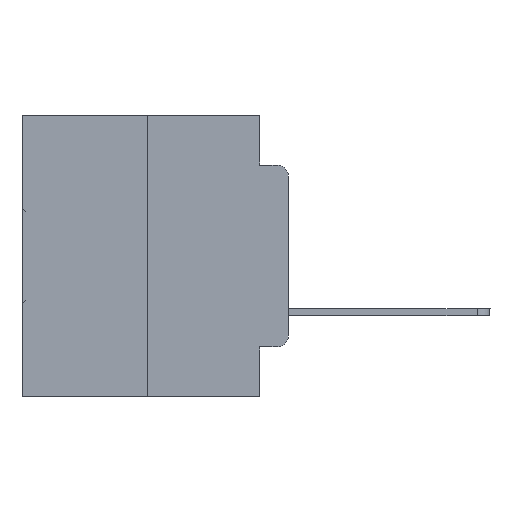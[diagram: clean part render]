
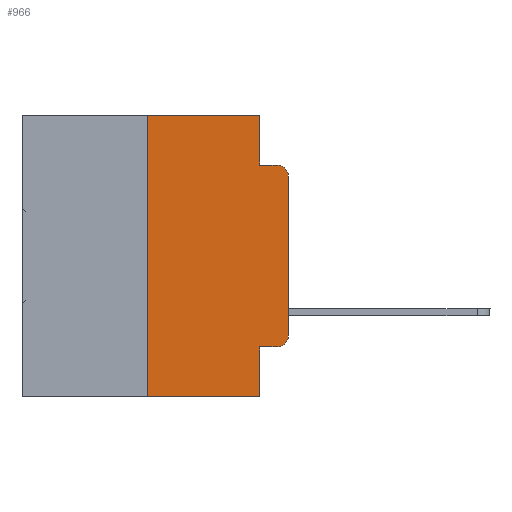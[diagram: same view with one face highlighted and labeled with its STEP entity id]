
A CAD part, left-side view. The second image highlights one B-rep face of the part: STEP entity #966.
In plain terms, the highlighted planar face has unit normal (-1, 0, 0).
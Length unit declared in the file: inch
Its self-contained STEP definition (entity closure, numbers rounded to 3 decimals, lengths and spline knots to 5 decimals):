
#112 = ORIENTED_EDGE ( 'NONE', *, *, #23995, .T. ) ;
#920 = VECTOR ( 'NONE', #23624, 39.37008 ) ;
#966 = ADVANCED_FACE ( 'NONE', ( #29396 ), #2952, .F. ) ;
#1161 = VECTOR ( 'NONE', #7430, 39.37008 ) ;
#1223 = VERTEX_POINT ( 'NONE', #29912 ) ;
#1409 = AXIS2_PLACEMENT_3D ( 'NONE', #13120, #25485, #3634 ) ;
#2000 = LINE ( 'NONE', #29377, #27557 ) ;
#2409 = CARTESIAN_POINT ( 'NONE',  ( 0., 0.25, 0. ) ) ;
#2458 = DIRECTION ( 'NONE',  ( -1., 0., 0. ) ) ;
#2721 = ORIENTED_EDGE ( 'NONE', *, *, #17437, .T. ) ;
#2754 = CARTESIAN_POINT ( 'NONE',  ( 0., 0.25, 0. ) ) ;
#2849 = CARTESIAN_POINT ( 'NONE',  ( 0., 0.473, 0. ) ) ;
#2899 = EDGE_CURVE ( 'NONE', #1223, #3802, #29334, .T. ) ;
#2952 = PLANE ( 'NONE',  #11335 ) ;
#3063 = DIRECTION ( 'NONE',  ( 0., 0., 1. ) ) ;
#3634 = DIRECTION ( 'NONE',  ( 0., 0., -1. ) ) ;
#3802 = VERTEX_POINT ( 'NONE', #2754 ) ;
#5614 = VERTEX_POINT ( 'NONE', #30076 ) ;
#6177 = EDGE_CURVE ( 'NONE', #16254, #25767, #12378, .T. ) ;
#6538 = CARTESIAN_POINT ( 'NONE',  ( 0., 0.051, -0.0885 ) ) ;
#7061 = LINE ( 'NONE', #28734, #12035 ) ;
#7262 = CARTESIAN_POINT ( 'NONE',  ( 0., 0.02, -0.3915 ) ) ;
#7430 = DIRECTION ( 'NONE',  ( 0., -1., 0. ) ) ;
#8000 = CARTESIAN_POINT ( 'NONE',  ( 0., 0., 0. ) ) ;
#9106 = EDGE_CURVE ( 'NONE', #31062, #9391, #9989, .T. ) ;
#9331 = ORIENTED_EDGE ( 'NONE', *, *, #30141, .F. ) ;
#9391 = VERTEX_POINT ( 'NONE', #18485 ) ;
#9632 = CARTESIAN_POINT ( 'NONE',  ( 0., 0., -0.3915 ) ) ;
#9983 = ORIENTED_EDGE ( 'NONE', *, *, #9106, .T. ) ;
#9989 = LINE ( 'NONE', #24395, #1161 ) ;
#10152 = DIRECTION ( 'NONE',  ( 0., 0., -1. ) ) ;
#11181 = CARTESIAN_POINT ( 'NONE',  ( 0., 0., -0.1085 ) ) ;
#11335 = AXIS2_PLACEMENT_3D ( 'NONE', #2849, #27047, #17357 ) ;
#11986 = VECTOR ( 'NONE', #27375, 39.37008 ) ;
#12035 = VECTOR ( 'NONE', #16607, 39.37008 ) ;
#12378 = CIRCLE ( 'NONE', #1409, 0.02 ) ;
#12832 = CARTESIAN_POINT ( 'NONE',  ( 0., 0.051, 0. ) ) ;
#12867 = ORIENTED_EDGE ( 'NONE', *, *, #2899, .F. ) ;
#12878 = CARTESIAN_POINT ( 'NONE',  ( 0., 0.051, 0. ) ) ;
#12962 = LINE ( 'NONE', #8000, #16401 ) ;
#13006 = CARTESIAN_POINT ( 'NONE',  ( 0., 0.473, 0. ) ) ;
#13120 = CARTESIAN_POINT ( 'NONE',  ( 0., 0.02, -0.1085 ) ) ;
#13848 = ORIENTED_EDGE ( 'NONE', *, *, #25305, .T. ) ;
#14674 = DIRECTION ( 'NONE',  ( 0., 0., 1. ) ) ;
#15008 = AXIS2_PLACEMENT_3D ( 'NONE', #7262, #2458, #24337 ) ;
#15818 = VERTEX_POINT ( 'NONE', #26516 ) ;
#16254 = VERTEX_POINT ( 'NONE', #11181 ) ;
#16401 = VECTOR ( 'NONE', #3063, 39.37008 ) ;
#16607 = DIRECTION ( 'NONE',  ( 0., 0., -1. ) ) ;
#16817 = CARTESIAN_POINT ( 'NONE',  ( 0., 0.02, -0.0885 ) ) ;
#17236 = DIRECTION ( 'NONE',  ( 0., -1., 0. ) ) ;
#17357 = DIRECTION ( 'NONE',  ( 0., 0., -1. ) ) ;
#17437 = EDGE_CURVE ( 'NONE', #9391, #30083, #25323, .T. ) ;
#18124 = VERTEX_POINT ( 'NONE', #12878 ) ;
#18485 = CARTESIAN_POINT ( 'NONE',  ( 0., 0.02, -0.4115 ) ) ;
#19222 = ORIENTED_EDGE ( 'NONE', *, *, #6177, .T. ) ;
#20436 = LINE ( 'NONE', #12832, #27624 ) ;
#20787 = LINE ( 'NONE', #13006, #11986 ) ;
#21011 = CARTESIAN_POINT ( 'NONE',  ( 0., 0.051, -0.4115 ) ) ;
#23624 = DIRECTION ( 'NONE',  ( 0., -1., 0. ) ) ;
#23995 = EDGE_CURVE ( 'NONE', #1223, #5614, #2000, .T. ) ;
#24337 = DIRECTION ( 'NONE',  ( 0., 0., -1. ) ) ;
#24392 = VECTOR ( 'NONE', #14674, 39.37008 ) ;
#24395 = CARTESIAN_POINT ( 'NONE',  ( 0., 0.051, -0.4115 ) ) ;
#24545 = ORIENTED_EDGE ( 'NONE', *, *, #29333, .F. ) ;
#25305 = EDGE_CURVE ( 'NONE', #30083, #16254, #12962, .T. ) ;
#25323 = CIRCLE ( 'NONE', #15008, 0.02 ) ;
#25485 = DIRECTION ( 'NONE',  ( -1., 0., 0. ) ) ;
#25767 = VERTEX_POINT ( 'NONE', #16817 ) ;
#26516 = CARTESIAN_POINT ( 'NONE',  ( 0., 0.051, -0.0885 ) ) ;
#27047 = DIRECTION ( 'NONE',  ( 1., 0., 0. ) ) ;
#27256 = LINE ( 'NONE', #6538, #920 ) ;
#27375 = DIRECTION ( 'NONE',  ( 0., -1., 0. ) ) ;
#27557 = VECTOR ( 'NONE', #17236, 39.37008 ) ;
#27624 = VECTOR ( 'NONE', #10152, 39.37008 ) ;
#28681 = EDGE_CURVE ( 'NONE', #18124, #15818, #7061, .T. ) ;
#28734 = CARTESIAN_POINT ( 'NONE',  ( 0., 0.051, 0. ) ) ;
#29333 = EDGE_CURVE ( 'NONE', #15818, #25767, #27256, .T. ) ;
#29334 = LINE ( 'NONE', #2409, #24392 ) ;
#29377 = CARTESIAN_POINT ( 'NONE',  ( 0., 0.473, -0.5 ) ) ;
#29396 = FACE_OUTER_BOUND ( 'NONE', #31573, .T. ) ;
#29471 = EDGE_CURVE ( 'NONE', #31062, #5614, #20436, .T. ) ;
#29912 = CARTESIAN_POINT ( 'NONE',  ( 0., 0.25, -0.5 ) ) ;
#30076 = CARTESIAN_POINT ( 'NONE',  ( 0., 0.051, -0.5 ) ) ;
#30083 = VERTEX_POINT ( 'NONE', #9632 ) ;
#30141 = EDGE_CURVE ( 'NONE', #3802, #18124, #20787, .T. ) ;
#30430 = ORIENTED_EDGE ( 'NONE', *, *, #28681, .F. ) ;
#30435 = ORIENTED_EDGE ( 'NONE', *, *, #29471, .F. ) ;
#31062 = VERTEX_POINT ( 'NONE', #21011 ) ;
#31573 = EDGE_LOOP ( 'NONE', ( #13848, #19222, #24545, #30430, #9331, #12867, #112, #30435, #9983, #2721 ) ) ;
